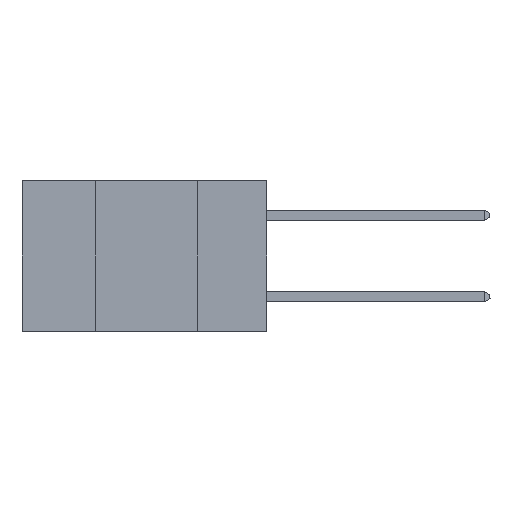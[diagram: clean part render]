
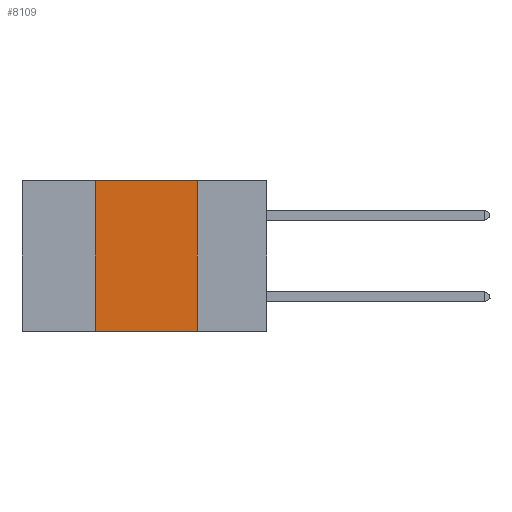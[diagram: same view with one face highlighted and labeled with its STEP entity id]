
A CAD part, left-side view. The second image highlights one B-rep face of the part: STEP entity #8109.
In plain terms, the highlighted planar face has unit normal (-1, 0, 0).
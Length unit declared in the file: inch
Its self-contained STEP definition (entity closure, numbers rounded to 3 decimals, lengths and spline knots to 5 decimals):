
#669 = CARTESIAN_POINT ( 'NONE',  ( 0., 0.42, 0. ) ) ;
#683 = CARTESIAN_POINT ( 'NONE',  ( 0., 0.6, 0. ) ) ;
#2087 = ORIENTED_EDGE ( 'NONE', *, *, #12276, .F. ) ;
#2218 = CARTESIAN_POINT ( 'NONE',  ( 0., 0.17, 0. ) ) ;
#2559 = FACE_OUTER_BOUND ( 'NONE', #3142, .T. ) ;
#2777 = EDGE_CURVE ( 'NONE', #10795, #16581, #13158, .T. ) ;
#3031 = DIRECTION ( 'NONE',  ( 0., -1., 0. ) ) ;
#3142 = EDGE_LOOP ( 'NONE', ( #5724, #2087, #13790, #10486 ) ) ;
#4189 = LINE ( 'NONE', #11856, #7264 ) ;
#4584 = LINE ( 'NONE', #10216, #11896 ) ;
#4911 = VECTOR ( 'NONE', #15327, 39.37008 ) ;
#5333 = DIRECTION ( 'NONE',  ( 1., 0., 0. ) ) ;
#5645 = CARTESIAN_POINT ( 'NONE',  ( 0., 0.42, -0.37 ) ) ;
#5724 = ORIENTED_EDGE ( 'NONE', *, *, #16365, .F. ) ;
#7264 = VECTOR ( 'NONE', #3031, 39.37008 ) ;
#8109 = ADVANCED_FACE ( 'NONE', ( #2559 ), #13936, .F. ) ;
#9258 = CARTESIAN_POINT ( 'NONE',  ( 0., 0.17, -0.37 ) ) ;
#9327 = LINE ( 'NONE', #2218, #4911 ) ;
#10216 = CARTESIAN_POINT ( 'NONE',  ( 0., 0.6, 0. ) ) ;
#10410 = VERTEX_POINT ( 'NONE', #9258 ) ;
#10429 = AXIS2_PLACEMENT_3D ( 'NONE', #683, #5333, #15320 ) ;
#10486 = ORIENTED_EDGE ( 'NONE', *, *, #16712, .T. ) ;
#10795 = VERTEX_POINT ( 'NONE', #5645 ) ;
#11450 = CARTESIAN_POINT ( 'NONE',  ( 0., 0.17, 0. ) ) ;
#11634 = DIRECTION ( 'NONE',  ( 0., -1., 0. ) ) ;
#11856 = CARTESIAN_POINT ( 'NONE',  ( 0., 0.6, -0.37 ) ) ;
#11896 = VECTOR ( 'NONE', #11634, 39.37008 ) ;
#12276 = EDGE_CURVE ( 'NONE', #16581, #17756, #4584, .T. ) ;
#12517 = DIRECTION ( 'NONE',  ( 0., 0., 1. ) ) ;
#12716 = VECTOR ( 'NONE', #12517, 39.37008 ) ;
#13158 = LINE ( 'NONE', #669, #12716 ) ;
#13790 = ORIENTED_EDGE ( 'NONE', *, *, #2777, .F. ) ;
#13936 = PLANE ( 'NONE',  #10429 ) ;
#15320 = DIRECTION ( 'NONE',  ( 0., 0., -1. ) ) ;
#15327 = DIRECTION ( 'NONE',  ( 0., 0., -1. ) ) ;
#16365 = EDGE_CURVE ( 'NONE', #17756, #10410, #9327, .T. ) ;
#16581 = VERTEX_POINT ( 'NONE', #18580 ) ;
#16712 = EDGE_CURVE ( 'NONE', #10795, #10410, #4189, .T. ) ;
#17756 = VERTEX_POINT ( 'NONE', #11450 ) ;
#18580 = CARTESIAN_POINT ( 'NONE',  ( 0., 0.42, 0. ) ) ;
